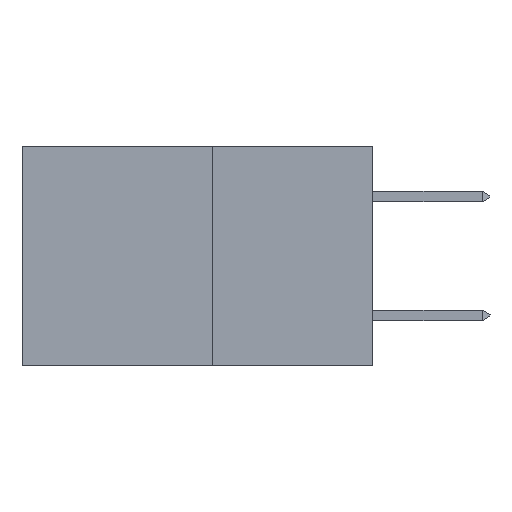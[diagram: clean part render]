
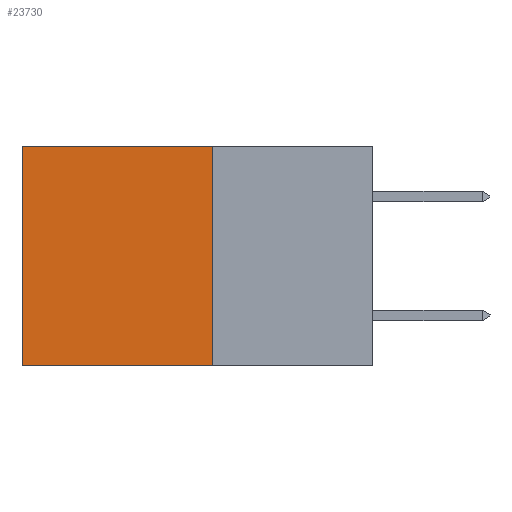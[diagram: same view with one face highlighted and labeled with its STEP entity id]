
A CAD part, left-side view. The second image highlights one B-rep face of the part: STEP entity #23730.
In plain terms, the highlighted planar face has unit normal (-1, 0, 0).
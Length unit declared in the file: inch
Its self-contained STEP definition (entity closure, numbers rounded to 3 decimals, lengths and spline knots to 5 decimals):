
#665 = LINE ( 'NONE', #15162, #20728 ) ;
#959 = CARTESIAN_POINT ( 'NONE',  ( 0.277, 0.59, 0. ) ) ;
#1589 = EDGE_CURVE ( 'NONE', #19217, #7275, #15346, .T. ) ;
#1794 = CARTESIAN_POINT ( 'NONE',  ( 0.277, 0.27, -0.37 ) ) ;
#2769 = EDGE_CURVE ( 'NONE', #13911, #22098, #665, .T. ) ;
#2841 = DIRECTION ( 'NONE',  ( 1., 0., 0. ) ) ;
#3683 = DIRECTION ( 'NONE',  ( 0., 0., -1. ) ) ;
#5342 = AXIS2_PLACEMENT_3D ( 'NONE', #12444, #2841, #16480 ) ;
#5430 = ORIENTED_EDGE ( 'NONE', *, *, #2769, .T. ) ;
#6466 = VECTOR ( 'NONE', #22849, 39.37008 ) ;
#6525 = DIRECTION ( 'NONE',  ( 0., 1., 0. ) ) ;
#6601 = CARTESIAN_POINT ( 'NONE',  ( 0.277, 0.27, -0.37 ) ) ;
#7095 = EDGE_CURVE ( 'NONE', #13911, #19217, #20792, .T. ) ;
#7123 = FACE_OUTER_BOUND ( 'NONE', #14670, .T. ) ;
#7275 = VERTEX_POINT ( 'NONE', #17539 ) ;
#7461 = CARTESIAN_POINT ( 'NONE',  ( 0.277, 0.59, -0.37 ) ) ;
#8296 = ORIENTED_EDGE ( 'NONE', *, *, #8487, .T. ) ;
#8487 = EDGE_CURVE ( 'NONE', #22098, #7275, #20724, .T. ) ;
#9126 = VECTOR ( 'NONE', #3683, 39.37008 ) ;
#11185 = CARTESIAN_POINT ( 'NONE',  ( 0.277, 0.27, -0.37 ) ) ;
#12444 = CARTESIAN_POINT ( 'NONE',  ( 0.277, 0.27, -0.37 ) ) ;
#13634 = ORIENTED_EDGE ( 'NONE', *, *, #7095, .F. ) ;
#13911 = VERTEX_POINT ( 'NONE', #18249 ) ;
#14670 = EDGE_LOOP ( 'NONE', ( #8296, #18707, #13634, #5430 ) ) ;
#15162 = CARTESIAN_POINT ( 'NONE',  ( 0.277, 0.27, 0. ) ) ;
#15189 = DIRECTION ( 'NONE',  ( 0., 1., 0. ) ) ;
#15346 = LINE ( 'NONE', #6601, #15973 ) ;
#15973 = VECTOR ( 'NONE', #6525, 39.37008 ) ;
#16480 = DIRECTION ( 'NONE',  ( 0., 0., -1. ) ) ;
#17539 = CARTESIAN_POINT ( 'NONE',  ( 0.277, 0.59, -0.37 ) ) ;
#18249 = CARTESIAN_POINT ( 'NONE',  ( 0.277, 0.27, 0. ) ) ;
#18707 = ORIENTED_EDGE ( 'NONE', *, *, #1589, .F. ) ;
#19217 = VERTEX_POINT ( 'NONE', #1794 ) ;
#20724 = LINE ( 'NONE', #7461, #9126 ) ;
#20728 = VECTOR ( 'NONE', #15189, 39.37008 ) ;
#20792 = LINE ( 'NONE', #11185, #6466 ) ;
#22098 = VERTEX_POINT ( 'NONE', #959 ) ;
#22849 = DIRECTION ( 'NONE',  ( 0., 0., -1. ) ) ;
#23730 = ADVANCED_FACE ( 'NONE', ( #7123 ), #24156, .F. ) ;
#24156 = PLANE ( 'NONE',  #5342 ) ;
